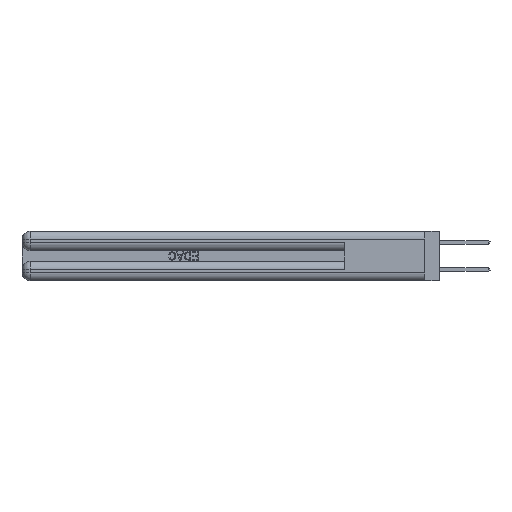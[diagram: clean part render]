
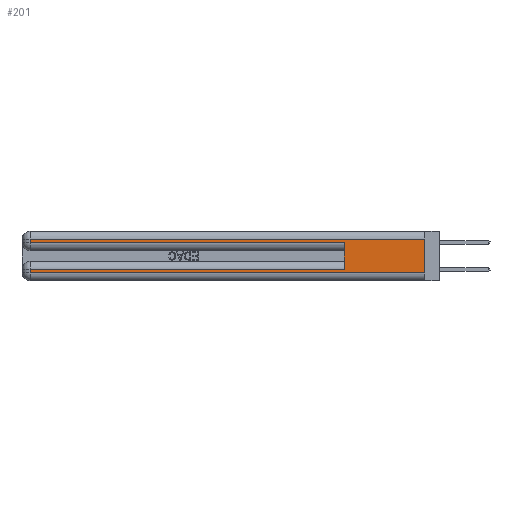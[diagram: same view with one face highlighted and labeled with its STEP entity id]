
A CAD part, left-side view. The second image highlights one B-rep face of the part: STEP entity #201.
In plain terms, the highlighted planar face has unit normal (-1, 0, 0).
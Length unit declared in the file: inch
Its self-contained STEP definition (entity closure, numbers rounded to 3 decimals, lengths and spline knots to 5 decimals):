
#201 = ADVANCED_FACE ( 'NONE', ( #26877 ), #5205, .F. ) ;
#454 = DIRECTION ( 'NONE',  ( 0., -1., 0. ) ) ;
#2348 = CARTESIAN_POINT ( 'NONE',  ( 0., 0., 0.37 ) ) ;
#3542 = VECTOR ( 'NONE', #3777, 39.37008 ) ;
#3777 = DIRECTION ( 'NONE',  ( 0., 0., 1. ) ) ;
#4932 = ORIENTED_EDGE ( 'NONE', *, *, #22189, .T. ) ;
#4937 = LINE ( 'NONE', #30855, #38054 ) ;
#5205 = PLANE ( 'NONE',  #31705 ) ;
#5209 = CARTESIAN_POINT ( 'NONE',  ( 0., 2.94, 0.37 ) ) ;
#6088 = VERTEX_POINT ( 'NONE', #34378 ) ;
#6187 = CARTESIAN_POINT ( 'NONE',  ( 0., 0.6, 0.085 ) ) ;
#6191 = CARTESIAN_POINT ( 'NONE',  ( 0., 2.94, 0.085 ) ) ;
#7381 = LINE ( 'NONE', #35067, #39523 ) ;
#7716 = VECTOR ( 'NONE', #27564, 39.37008 ) ;
#7779 = DIRECTION ( 'NONE',  ( 0., -1., 0. ) ) ;
#7829 = VECTOR ( 'NONE', #454, 39.37008 ) ;
#8410 = DIRECTION ( 'NONE',  ( 0., 0., -1. ) ) ;
#8780 = LINE ( 'NONE', #5209, #16315 ) ;
#9558 = VERTEX_POINT ( 'NONE', #6187 ) ;
#9560 = CARTESIAN_POINT ( 'NONE',  ( 0., 0.6, 0.285 ) ) ;
#10187 = CARTESIAN_POINT ( 'NONE',  ( 0., 0.6, 0.145 ) ) ;
#10270 = CARTESIAN_POINT ( 'NONE',  ( 0., 0., 0.31 ) ) ;
#11620 = DIRECTION ( 'NONE',  ( 0., 0., -1. ) ) ;
#12762 = EDGE_CURVE ( 'NONE', #9558, #38400, #20651, .T. ) ;
#13474 = EDGE_CURVE ( 'NONE', #6088, #35496, #20654, .T. ) ;
#14733 = CARTESIAN_POINT ( 'NONE',  ( 0., 0., 0.085 ) ) ;
#15808 = DIRECTION ( 'NONE',  ( 0., 1., 0. ) ) ;
#16315 = VECTOR ( 'NONE', #8410, 39.37008 ) ;
#16356 = LINE ( 'NONE', #16447, #7829 ) ;
#16447 = CARTESIAN_POINT ( 'NONE',  ( 0., 0., 0.285 ) ) ;
#16743 = ORIENTED_EDGE ( 'NONE', *, *, #20178, .T. ) ;
#17322 = CARTESIAN_POINT ( 'NONE',  ( 0., 0., 0.06 ) ) ;
#17642 = ORIENTED_EDGE ( 'NONE', *, *, #29381, .T. ) ;
#18650 = VERTEX_POINT ( 'NONE', #35099 ) ;
#20024 = CARTESIAN_POINT ( 'NONE',  ( 0., 2.94, 0.285 ) ) ;
#20178 = EDGE_CURVE ( 'NONE', #38375, #6088, #4937, .T. ) ;
#20427 = VERTEX_POINT ( 'NONE', #10270 ) ;
#20651 = LINE ( 'NONE', #10187, #3542 ) ;
#20654 = LINE ( 'NONE', #17322, #38714 ) ;
#21518 = EDGE_CURVE ( 'NONE', #20427, #18650, #7381, .T. ) ;
#22189 = EDGE_CURVE ( 'NONE', #30448, #38400, #16356, .T. ) ;
#23311 = EDGE_LOOP ( 'NONE', ( #28301, #25617, #17642, #4932, #31945, #33659, #16743, #25130 ) ) ;
#24859 = DIRECTION ( 'NONE',  ( 0., 0., -1. ) ) ;
#25130 = ORIENTED_EDGE ( 'NONE', *, *, #13474, .T. ) ;
#25617 = ORIENTED_EDGE ( 'NONE', *, *, #21518, .T. ) ;
#26877 = FACE_OUTER_BOUND ( 'NONE', #23311, .T. ) ;
#27564 = DIRECTION ( 'NONE',  ( 0., 1., 0. ) ) ;
#27649 = VECTOR ( 'NONE', #24859, 39.37008 ) ;
#27691 = CARTESIAN_POINT ( 'NONE',  ( 0., 0., 0.37 ) ) ;
#28301 = ORIENTED_EDGE ( 'NONE', *, *, #35123, .F. ) ;
#28672 = LINE ( 'NONE', #2348, #27649 ) ;
#29381 = EDGE_CURVE ( 'NONE', #18650, #30448, #8780, .T. ) ;
#30448 = VERTEX_POINT ( 'NONE', #20024 ) ;
#30855 = CARTESIAN_POINT ( 'NONE',  ( 0., 2.94, 0.37 ) ) ;
#30927 = DIRECTION ( 'NONE',  ( 1., 0., 0. ) ) ;
#31357 = LINE ( 'NONE', #14733, #7716 ) ;
#31705 = AXIS2_PLACEMENT_3D ( 'NONE', #27691, #30927, #11620 ) ;
#31945 = ORIENTED_EDGE ( 'NONE', *, *, #12762, .F. ) ;
#33659 = ORIENTED_EDGE ( 'NONE', *, *, #38674, .T. ) ;
#34066 = DIRECTION ( 'NONE',  ( 0., 0., -1. ) ) ;
#34378 = CARTESIAN_POINT ( 'NONE',  ( 0., 2.94, 0.06 ) ) ;
#35067 = CARTESIAN_POINT ( 'NONE',  ( 0., 0., 0.31 ) ) ;
#35099 = CARTESIAN_POINT ( 'NONE',  ( 0., 2.94, 0.31 ) ) ;
#35123 = EDGE_CURVE ( 'NONE', #20427, #35496, #28672, .T. ) ;
#35496 = VERTEX_POINT ( 'NONE', #39661 ) ;
#38054 = VECTOR ( 'NONE', #34066, 39.37008 ) ;
#38375 = VERTEX_POINT ( 'NONE', #6191 ) ;
#38400 = VERTEX_POINT ( 'NONE', #9560 ) ;
#38674 = EDGE_CURVE ( 'NONE', #9558, #38375, #31357, .T. ) ;
#38714 = VECTOR ( 'NONE', #7779, 39.37008 ) ;
#39523 = VECTOR ( 'NONE', #15808, 39.37008 ) ;
#39661 = CARTESIAN_POINT ( 'NONE',  ( 0., 0., 0.06 ) ) ;
